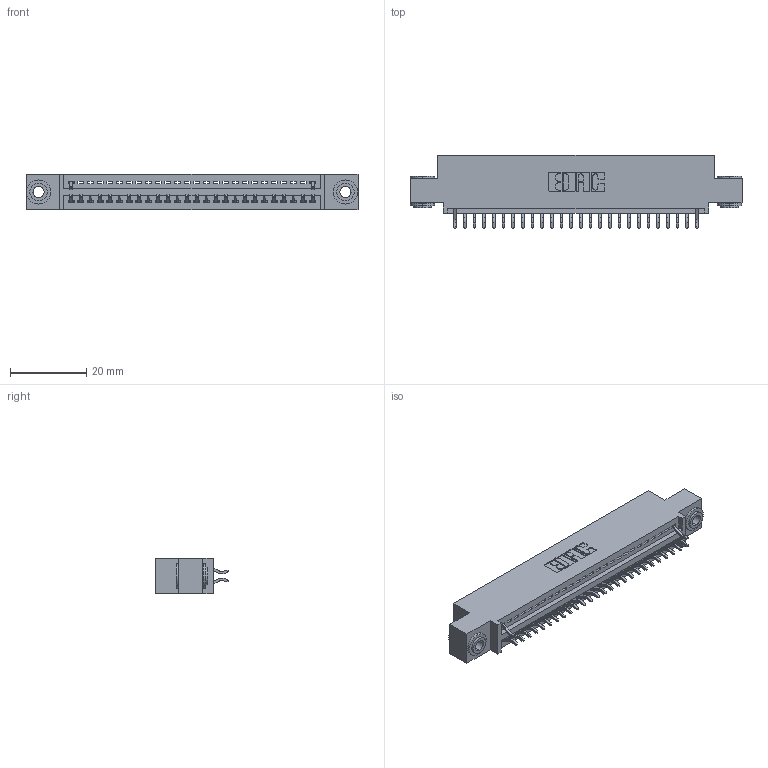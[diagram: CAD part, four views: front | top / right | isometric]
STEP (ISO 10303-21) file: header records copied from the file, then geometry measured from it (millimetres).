
FILE_DESCRIPTION (( 'STEP AP203' ), '1' );
FILE_NAME ('345-052-556-503.STEP', '2018-09-22T23:58:11', ( '' ), ( '' ), 'SwSTEP 2.0', 'SolidWorks 2016', '' );
FILE_SCHEMA (( 'CONFIG_CONTROL_DESIGN' ));
Length unit declared in the file: inch
Products named in the file (4): 345-292-001_556 Tail; 345-250-002_345-250-002-102; 345-052-556-503; 345 Part_0.110 Offset - 0.156 Dia-TH
Assembly tree (31 placements, depth 2):
  345-052-556-503
    345 Part_0.110 Offset - 0.156 Dia-TH
    345-292-001_556 Tail  x28
    345-250-002_345-250-002-102  x2
Bounding box: 87.25 x 19.24 x 9.4 mm (x, y, z)
Volume: 8055.5 mm3; surface area: 10645.4 mm2
Topology: 31 solids, 31 shells, 1928 faces, 5753 edges, 3794 vertices
Faces by surface type: plane 1298, cylinder 622, cone 8
Entity records: 22788 total; most frequent: CARTESIAN_POINT 3931, ORIENTED_EDGE 3870, DIRECTION 3477, EDGE_CURVE 1935, VECTOR 1667, LINE 1667, VERTEX_POINT 1286, AXIS2_PLACEMENT_3D 905
